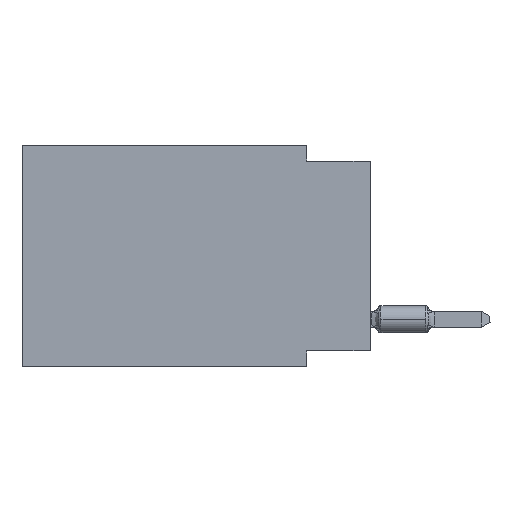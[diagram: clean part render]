
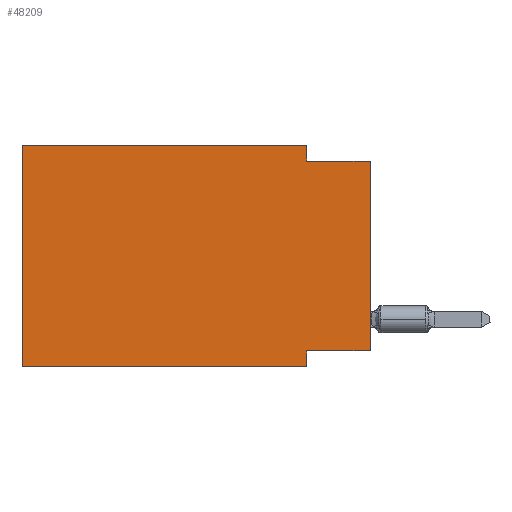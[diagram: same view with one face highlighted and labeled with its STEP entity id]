
A CAD part, left-side view. The second image highlights one B-rep face of the part: STEP entity #48209.
In plain terms, the highlighted planar face has unit normal (-1, 0, 0).
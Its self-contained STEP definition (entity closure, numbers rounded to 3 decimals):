
#194 = VECTOR ( 'NONE', #22508, 1000. ) ;
#576 = VERTEX_POINT ( 'NONE', #20794 ) ;
#1463 = EDGE_CURVE ( 'NONE', #576, #30059, #44669, .T. ) ;
#2235 = LINE ( 'NONE', #15574, #6942 ) ;
#2403 = VERTEX_POINT ( 'NONE', #9921 ) ;
#4612 = DIRECTION ( 'NONE',  ( 0., 0., -1. ) ) ;
#5327 = ORIENTED_EDGE ( 'NONE', *, *, #19947, .T. ) ;
#6168 = DIRECTION ( 'NONE',  ( 0., 0., 1. ) ) ;
#6716 = LINE ( 'NONE', #33962, #45632 ) ;
#6919 = VECTOR ( 'NONE', #11653, 1000. ) ;
#6925 = EDGE_CURVE ( 'NONE', #29818, #45659, #9416, .T. ) ;
#6942 = VECTOR ( 'NONE', #6168, 1000. ) ;
#8549 = LINE ( 'NONE', #41819, #11777 ) ;
#8594 = CARTESIAN_POINT ( 'NONE',  ( 0., 0., -0.635 ) ) ;
#9416 = LINE ( 'NONE', #27880, #32558 ) ;
#9921 = CARTESIAN_POINT ( 'NONE',  ( 0., 2.54, -8.89 ) ) ;
#10151 = CARTESIAN_POINT ( 'NONE',  ( 0., 0., -0.635 ) ) ;
#10429 = EDGE_CURVE ( 'NONE', #45659, #23390, #8549, .T. ) ;
#10694 = EDGE_CURVE ( 'NONE', #30059, #2403, #12140, .T. ) ;
#11387 = VERTEX_POINT ( 'NONE', #43108 ) ;
#11653 = DIRECTION ( 'NONE',  ( 0., -1., 0. ) ) ;
#11777 = VECTOR ( 'NONE', #4612, 1000. ) ;
#12140 = LINE ( 'NONE', #26350, #18394 ) ;
#12846 = LINE ( 'NONE', #8594, #194 ) ;
#15574 = CARTESIAN_POINT ( 'NONE',  ( 0., 13.97, 0. ) ) ;
#16799 = AXIS2_PLACEMENT_3D ( 'NONE', #33368, #47912, #47621 ) ;
#18394 = VECTOR ( 'NONE', #58143, 1000. ) ;
#18396 = ORIENTED_EDGE ( 'NONE', *, *, #10429, .F. ) ;
#19635 = EDGE_CURVE ( 'NONE', #11387, #2403, #40638, .T. ) ;
#19947 = EDGE_CURVE ( 'NONE', #576, #21766, #6716, .T. ) ;
#20794 = CARTESIAN_POINT ( 'NONE',  ( 0., 0., -8.255 ) ) ;
#21051 = ORIENTED_EDGE ( 'NONE', *, *, #58788, .F. ) ;
#21766 = VERTEX_POINT ( 'NONE', #10151 ) ;
#22508 = DIRECTION ( 'NONE',  ( 0., -1., 0. ) ) ;
#23390 = VERTEX_POINT ( 'NONE', #53149 ) ;
#24305 = PLANE ( 'NONE',  #16799 ) ;
#25229 = ORIENTED_EDGE ( 'NONE', *, *, #6925, .F. ) ;
#25910 = CARTESIAN_POINT ( 'NONE',  ( 0., 0., -8.255 ) ) ;
#26350 = CARTESIAN_POINT ( 'NONE',  ( 0., 2.54, -8.89 ) ) ;
#27260 = VECTOR ( 'NONE', #58574, 1000. ) ;
#27880 = CARTESIAN_POINT ( 'NONE',  ( 0., 13.97, 0. ) ) ;
#28127 = CARTESIAN_POINT ( 'NONE',  ( 0., 13.97, 0. ) ) ;
#29440 = FACE_OUTER_BOUND ( 'NONE', #55434, .T. ) ;
#29818 = VERTEX_POINT ( 'NONE', #28127 ) ;
#30059 = VERTEX_POINT ( 'NONE', #58050 ) ;
#32558 = VECTOR ( 'NONE', #58607, 1000. ) ;
#33348 = DIRECTION ( 'NONE',  ( 0., 0., 1. ) ) ;
#33368 = CARTESIAN_POINT ( 'NONE',  ( 0., 13.97, 0. ) ) ;
#33962 = CARTESIAN_POINT ( 'NONE',  ( 0., 0., 0. ) ) ;
#36944 = ORIENTED_EDGE ( 'NONE', *, *, #10694, .F. ) ;
#40638 = LINE ( 'NONE', #53987, #6919 ) ;
#41819 = CARTESIAN_POINT ( 'NONE',  ( 0., 2.54, 0. ) ) ;
#43108 = CARTESIAN_POINT ( 'NONE',  ( 0., 13.97, -8.89 ) ) ;
#44669 = LINE ( 'NONE', #25910, #27260 ) ;
#44922 = ORIENTED_EDGE ( 'NONE', *, *, #19635, .T. ) ;
#45503 = CARTESIAN_POINT ( 'NONE',  ( 0., 2.54, 0. ) ) ;
#45632 = VECTOR ( 'NONE', #33348, 1000. ) ;
#45659 = VERTEX_POINT ( 'NONE', #45503 ) ;
#46256 = ORIENTED_EDGE ( 'NONE', *, *, #1463, .F. ) ;
#47621 = DIRECTION ( 'NONE',  ( 0., 0., -1. ) ) ;
#47912 = DIRECTION ( 'NONE',  ( 1., 0., 0. ) ) ;
#48209 = ADVANCED_FACE ( 'NONE', ( #29440 ), #24305, .F. ) ;
#50831 = EDGE_CURVE ( 'NONE', #11387, #29818, #2235, .T. ) ;
#53149 = CARTESIAN_POINT ( 'NONE',  ( 0., 2.54, -0.635 ) ) ;
#53987 = CARTESIAN_POINT ( 'NONE',  ( 0., 13.97, -8.89 ) ) ;
#55434 = EDGE_LOOP ( 'NONE', ( #5327, #21051, #18396, #25229, #57643, #44922, #36944, #46256 ) ) ;
#57643 = ORIENTED_EDGE ( 'NONE', *, *, #50831, .F. ) ;
#58050 = CARTESIAN_POINT ( 'NONE',  ( 0., 2.54, -8.255 ) ) ;
#58143 = DIRECTION ( 'NONE',  ( 0., 0., -1. ) ) ;
#58574 = DIRECTION ( 'NONE',  ( 0., 1., 0. ) ) ;
#58607 = DIRECTION ( 'NONE',  ( 0., -1., 0. ) ) ;
#58788 = EDGE_CURVE ( 'NONE', #23390, #21766, #12846, .T. ) ;
